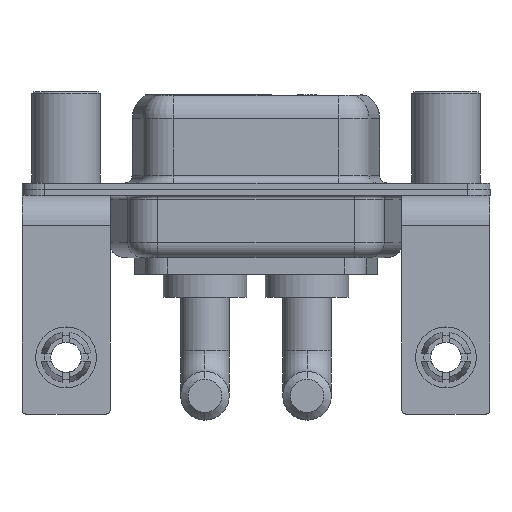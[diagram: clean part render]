
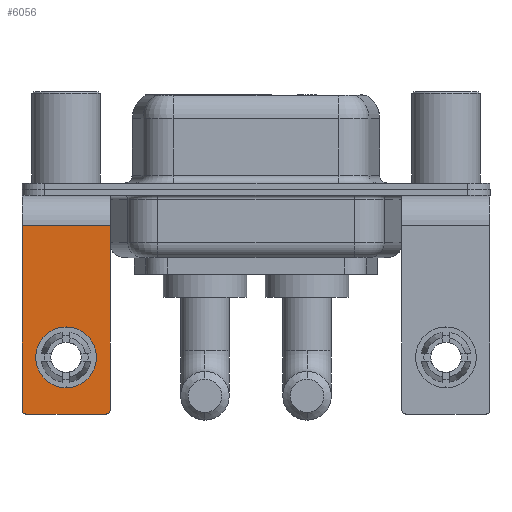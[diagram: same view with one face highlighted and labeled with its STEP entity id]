
A CAD part, front view. The second image highlights one B-rep face of the part: STEP entity #6056.
In plain terms, the highlighted planar face has unit normal (0, -1, 0).
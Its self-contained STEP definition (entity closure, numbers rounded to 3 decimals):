
#134 = LINE ( 'NONE', #10447, #9144 ) ;
#259 = DIRECTION ( 'NONE',  ( 0., 0., -1. ) ) ;
#350 = EDGE_CURVE ( 'NONE', #2778, #13158, #4634, .T. ) ;
#694 = LINE ( 'NONE', #8120, #10503 ) ;
#1197 = AXIS2_PLACEMENT_3D ( 'NONE', #6887, #11917, #10543 ) ;
#1221 = EDGE_CURVE ( 'NONE', #10391, #8681, #9631, .T. ) ;
#1673 = LINE ( 'NONE', #6968, #12407 ) ;
#1733 = CIRCLE ( 'NONE', #4744, 0.25 ) ;
#1770 = CARTESIAN_POINT ( 'NONE',  ( 2.9, -6.25, -2.4 ) ) ;
#2187 = ORIENTED_EDGE ( 'NONE', *, *, #350, .T. ) ;
#2778 = VERTEX_POINT ( 'NONE', #10735 ) ;
#2842 = EDGE_LOOP ( 'NONE', ( #13099, #12384, #4407, #10304, #12480, #15013 ) ) ;
#2969 = AXIS2_PLACEMENT_3D ( 'NONE', #5412, #5237, #11823 ) ;
#3644 = CIRCLE ( 'NONE', #1197, 0.25 ) ;
#3723 = CARTESIAN_POINT ( 'NONE',  ( 2.9, -6.25, -2.4 ) ) ;
#3880 = DIRECTION ( 'NONE',  ( 0., -1., 0. ) ) ;
#4407 = ORIENTED_EDGE ( 'NONE', *, *, #12574, .F. ) ;
#4634 = CIRCLE ( 'NONE', #15814, 2. ) ;
#4744 = AXIS2_PLACEMENT_3D ( 'NONE', #15411, #3880, #6546 ) ;
#5237 = DIRECTION ( 'NONE',  ( 0., 1., 0. ) ) ;
#5412 = CARTESIAN_POINT ( 'NONE',  ( 0., -6.25, -11.07 ) ) ;
#5818 = ORIENTED_EDGE ( 'NONE', *, *, #16042, .T. ) ;
#5910 = CARTESIAN_POINT ( 'NONE',  ( 0., -6.25, -11.07 ) ) ;
#6056 = ADVANCED_FACE ( 'NONE', ( #8505, #12263 ), #12339, .F. ) ;
#6074 = CARTESIAN_POINT ( 'NONE',  ( -2.9, -6.25, -2.4 ) ) ;
#6163 = DIRECTION ( 'NONE',  ( 0., 0., 1. ) ) ;
#6546 = DIRECTION ( 'NONE',  ( 0., 0., 1. ) ) ;
#6579 = CARTESIAN_POINT ( 'NONE',  ( -2.65, -6.25, -14.8 ) ) ;
#6887 = CARTESIAN_POINT ( 'NONE',  ( 2.65, -6.25, -14.55 ) ) ;
#6968 = CARTESIAN_POINT ( 'NONE',  ( 2.9, -6.25, -2.4 ) ) ;
#7158 = VECTOR ( 'NONE', #259, 1000. ) ;
#7710 = EDGE_CURVE ( 'NONE', #9985, #8115, #134, .T. ) ;
#7925 = VERTEX_POINT ( 'NONE', #12892 ) ;
#8115 = VERTEX_POINT ( 'NONE', #10933 ) ;
#8120 = CARTESIAN_POINT ( 'NONE',  ( 2.9, -6.25, -14.8 ) ) ;
#8399 = DIRECTION ( 'NONE',  ( 0., 0., -1. ) ) ;
#8505 = FACE_BOUND ( 'NONE', #12455, .T. ) ;
#8681 = VERTEX_POINT ( 'NONE', #16018 ) ;
#9106 = EDGE_CURVE ( 'NONE', #7925, #8681, #3644, .T. ) ;
#9144 = VECTOR ( 'NONE', #8399, 1000. ) ;
#9631 = LINE ( 'NONE', #10745, #7158 ) ;
#9985 = VERTEX_POINT ( 'NONE', #6074 ) ;
#10304 = ORIENTED_EDGE ( 'NONE', *, *, #9106, .T. ) ;
#10331 = EDGE_CURVE ( 'NONE', #8115, #15026, #1733, .T. ) ;
#10391 = VERTEX_POINT ( 'NONE', #3723 ) ;
#10447 = CARTESIAN_POINT ( 'NONE',  ( -2.9, -6.25, -2.4 ) ) ;
#10503 = VECTOR ( 'NONE', #12540, 1000. ) ;
#10543 = DIRECTION ( 'NONE',  ( 0., 0., 1. ) ) ;
#10735 = CARTESIAN_POINT ( 'NONE',  ( 0., -6.25, -13.07 ) ) ;
#10745 = CARTESIAN_POINT ( 'NONE',  ( 2.9, -6.25, -2.4 ) ) ;
#10933 = CARTESIAN_POINT ( 'NONE',  ( -2.9, -6.25, -14.55 ) ) ;
#11823 = DIRECTION ( 'NONE',  ( 0., 0., 1. ) ) ;
#11917 = DIRECTION ( 'NONE',  ( 0., -1., 0. ) ) ;
#12263 = FACE_OUTER_BOUND ( 'NONE', #2842, .T. ) ;
#12339 = PLANE ( 'NONE',  #14583 ) ;
#12384 = ORIENTED_EDGE ( 'NONE', *, *, #10331, .T. ) ;
#12407 = VECTOR ( 'NONE', #15646, 1000. ) ;
#12455 = EDGE_LOOP ( 'NONE', ( #2187, #5818 ) ) ;
#12480 = ORIENTED_EDGE ( 'NONE', *, *, #1221, .F. ) ;
#12540 = DIRECTION ( 'NONE',  ( -1., 0., 0. ) ) ;
#12574 = EDGE_CURVE ( 'NONE', #7925, #15026, #694, .T. ) ;
#12726 = EDGE_CURVE ( 'NONE', #10391, #9985, #1673, .T. ) ;
#12892 = CARTESIAN_POINT ( 'NONE',  ( 2.65, -6.25, -14.8 ) ) ;
#13001 = CARTESIAN_POINT ( 'NONE',  ( 0., -6.25, -9.07 ) ) ;
#13099 = ORIENTED_EDGE ( 'NONE', *, *, #7710, .T. ) ;
#13158 = VERTEX_POINT ( 'NONE', #13001 ) ;
#13371 = DIRECTION ( 'NONE',  ( 0., 1., 0. ) ) ;
#13696 = DIRECTION ( 'NONE',  ( 0., 0., 1. ) ) ;
#13923 = DIRECTION ( 'NONE',  ( 0., 1., 0. ) ) ;
#14583 = AXIS2_PLACEMENT_3D ( 'NONE', #1770, #13371, #13696 ) ;
#15013 = ORIENTED_EDGE ( 'NONE', *, *, #12726, .T. ) ;
#15026 = VERTEX_POINT ( 'NONE', #6579 ) ;
#15411 = CARTESIAN_POINT ( 'NONE',  ( -2.65, -6.25, -14.55 ) ) ;
#15646 = DIRECTION ( 'NONE',  ( -1., 0., 0. ) ) ;
#15814 = AXIS2_PLACEMENT_3D ( 'NONE', #5910, #13923, #6163 ) ;
#16018 = CARTESIAN_POINT ( 'NONE',  ( 2.9, -6.25, -14.55 ) ) ;
#16042 = EDGE_CURVE ( 'NONE', #13158, #2778, #16580, .T. ) ;
#16580 = CIRCLE ( 'NONE', #2969, 2. ) ;
